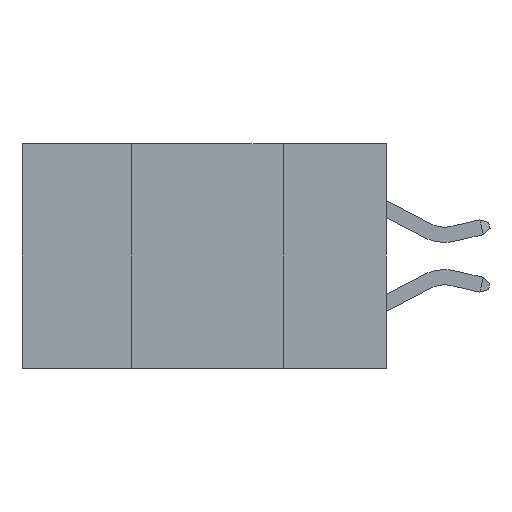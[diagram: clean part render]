
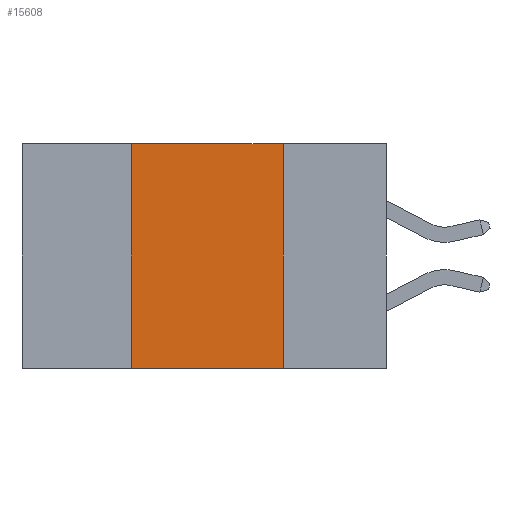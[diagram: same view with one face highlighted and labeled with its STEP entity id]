
A CAD part, left-side view. The second image highlights one B-rep face of the part: STEP entity #15608.
In plain terms, the highlighted planar face has unit normal (-1, 0, 0).
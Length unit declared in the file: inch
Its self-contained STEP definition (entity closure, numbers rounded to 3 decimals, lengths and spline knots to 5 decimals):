
#1310 = LINE ( 'NONE', #14768, #24770 ) ;
#2578 = CARTESIAN_POINT ( 'NONE',  ( 0., 0.17, -0.37 ) ) ;
#2648 = VERTEX_POINT ( 'NONE', #2578 ) ;
#4781 = VERTEX_POINT ( 'NONE', #11602 ) ;
#5968 = DIRECTION ( 'NONE',  ( 0., -1., 0. ) ) ;
#7098 = VERTEX_POINT ( 'NONE', #20586 ) ;
#7568 = AXIS2_PLACEMENT_3D ( 'NONE', #7736, #24064, #10089 ) ;
#7736 = CARTESIAN_POINT ( 'NONE',  ( 0., 0.6, 0. ) ) ;
#7791 = DIRECTION ( 'NONE',  ( 0., -1., 0. ) ) ;
#9926 = ORIENTED_EDGE ( 'NONE', *, *, #11329, .F. ) ;
#10089 = DIRECTION ( 'NONE',  ( 0., 0., -1. ) ) ;
#11329 = EDGE_CURVE ( 'NONE', #4781, #2648, #15056, .T. ) ;
#11602 = CARTESIAN_POINT ( 'NONE',  ( 0., 0.17, 0. ) ) ;
#11669 = VECTOR ( 'NONE', #26976, 39.37008 ) ;
#11789 = CARTESIAN_POINT ( 'NONE',  ( 0., 0.17, 0. ) ) ;
#12403 = LINE ( 'NONE', #24536, #11669 ) ;
#14514 = ORIENTED_EDGE ( 'NONE', *, *, #29044, .T. ) ;
#14768 = CARTESIAN_POINT ( 'NONE',  ( 0., 0.6, 0. ) ) ;
#15056 = LINE ( 'NONE', #11789, #15770 ) ;
#15608 = ADVANCED_FACE ( 'NONE', ( #17519 ), #19396, .F. ) ;
#15770 = VECTOR ( 'NONE', #28064, 39.37008 ) ;
#15773 = EDGE_LOOP ( 'NONE', ( #9926, #17647, #19080, #14514 ) ) ;
#17519 = FACE_OUTER_BOUND ( 'NONE', #15773, .T. ) ;
#17647 = ORIENTED_EDGE ( 'NONE', *, *, #30146, .F. ) ;
#19080 = ORIENTED_EDGE ( 'NONE', *, *, #22849, .F. ) ;
#19396 = PLANE ( 'NONE',  #7568 ) ;
#20172 = CARTESIAN_POINT ( 'NONE',  ( 0., 0.42, -0.37 ) ) ;
#20586 = CARTESIAN_POINT ( 'NONE',  ( 0., 0.42, 0. ) ) ;
#22849 = EDGE_CURVE ( 'NONE', #24866, #7098, #12403, .T. ) ;
#24064 = DIRECTION ( 'NONE',  ( 1., 0., 0. ) ) ;
#24536 = CARTESIAN_POINT ( 'NONE',  ( 0., 0.42, 0. ) ) ;
#24770 = VECTOR ( 'NONE', #7791, 39.37008 ) ;
#24866 = VERTEX_POINT ( 'NONE', #20172 ) ;
#25208 = VECTOR ( 'NONE', #5968, 39.37008 ) ;
#25930 = LINE ( 'NONE', #26912, #25208 ) ;
#26912 = CARTESIAN_POINT ( 'NONE',  ( 0., 0.6, -0.37 ) ) ;
#26976 = DIRECTION ( 'NONE',  ( 0., 0., 1. ) ) ;
#28064 = DIRECTION ( 'NONE',  ( 0., 0., -1. ) ) ;
#29044 = EDGE_CURVE ( 'NONE', #24866, #2648, #25930, .T. ) ;
#30146 = EDGE_CURVE ( 'NONE', #7098, #4781, #1310, .T. ) ;
